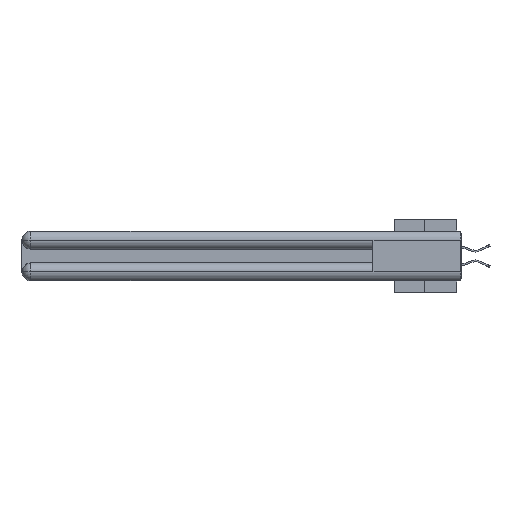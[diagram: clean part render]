
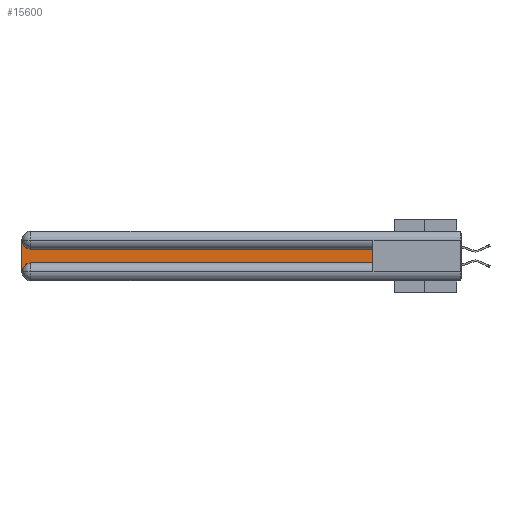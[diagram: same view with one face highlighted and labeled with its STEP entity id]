
A CAD part, left-side view. The second image highlights one B-rep face of the part: STEP entity #15600.
In plain terms, the highlighted planar face has unit normal (-1, 0, 0).
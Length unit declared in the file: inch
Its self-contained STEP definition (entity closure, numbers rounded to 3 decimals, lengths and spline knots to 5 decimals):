
#283 = VERTEX_POINT ( 'NONE', #14710 ) ;
#339 = EDGE_CURVE ( 'NONE', #48209, #17066, #15522, .T. ) ;
#643 = DIRECTION ( 'NONE',  ( 0., 0., -1. ) ) ;
#1827 = AXIS2_PLACEMENT_3D ( 'NONE', #17533, #47625, #32470 ) ;
#1992 = CARTESIAN_POINT ( 'NONE',  ( 0.075, 3., -0.0625 ) ) ;
#3666 = CARTESIAN_POINT ( 'NONE',  ( 0.075, 2.94, -0.2175 ) ) ;
#3961 = VERTEX_POINT ( 'NONE', #3666 ) ;
#4577 = CARTESIAN_POINT ( 'NONE',  ( 0.075, 0.6, -0.2175 ) ) ;
#4660 = CARTESIAN_POINT ( 'NONE',  ( 0.075, 0.6, -0.2175 ) ) ;
#5482 = EDGE_CURVE ( 'NONE', #17066, #39747, #42994, .T. ) ;
#9523 = ORIENTED_EDGE ( 'NONE', *, *, #43273, .T. ) ;
#11518 = DIRECTION ( 'NONE',  ( 1., 0., 0. ) ) ;
#12419 = FACE_OUTER_BOUND ( 'NONE', #30139, .T. ) ;
#13751 = VERTEX_POINT ( 'NONE', #4577 ) ;
#14710 = CARTESIAN_POINT ( 'NONE',  ( 0.075, 0.6, -0.1225 ) ) ;
#15522 = CIRCLE ( 'NONE', #20609, 0.06 ) ;
#15600 = ADVANCED_FACE ( 'NONE', ( #12419 ), #43793, .F. ) ;
#15812 = DIRECTION ( 'NONE',  ( 0., 0., 1. ) ) ;
#17066 = VERTEX_POINT ( 'NONE', #1992 ) ;
#17236 = ORIENTED_EDGE ( 'NONE', *, *, #18871, .T. ) ;
#17533 = CARTESIAN_POINT ( 'NONE',  ( 0.075, 3., -0.1225 ) ) ;
#17558 = CARTESIAN_POINT ( 'NONE',  ( 0.075, 2.94, -0.2775 ) ) ;
#18030 = VECTOR ( 'NONE', #48826, 39.37008 ) ;
#18871 = EDGE_CURVE ( 'NONE', #39747, #3961, #21706, .T. ) ;
#19211 = ORIENTED_EDGE ( 'NONE', *, *, #339, .T. ) ;
#20609 = AXIS2_PLACEMENT_3D ( 'NONE', #34315, #11518, #41828 ) ;
#21706 = CIRCLE ( 'NONE', #27857, 0.06 ) ;
#22790 = VECTOR ( 'NONE', #42804, 39.37008 ) ;
#25052 = DIRECTION ( 'NONE',  ( 0., 0., -1. ) ) ;
#26138 = EDGE_CURVE ( 'NONE', #3961, #13751, #32884, .T. ) ;
#27857 = AXIS2_PLACEMENT_3D ( 'NONE', #17558, #40153, #25052 ) ;
#27937 = CARTESIAN_POINT ( 'NONE',  ( 0.075, 2.94, -0.1225 ) ) ;
#29677 = ORIENTED_EDGE ( 'NONE', *, *, #26138, .T. ) ;
#30139 = EDGE_LOOP ( 'NONE', ( #31979, #19211, #46599, #17236, #29677, #9523 ) ) ;
#31979 = ORIENTED_EDGE ( 'NONE', *, *, #33174, .T. ) ;
#32470 = DIRECTION ( 'NONE',  ( 0., 0., -1. ) ) ;
#32848 = VECTOR ( 'NONE', #643, 39.37008 ) ;
#32884 = LINE ( 'NONE', #38951, #22790 ) ;
#33174 = EDGE_CURVE ( 'NONE', #283, #48209, #38227, .T. ) ;
#34315 = CARTESIAN_POINT ( 'NONE',  ( 0.075, 2.94, -0.0625 ) ) ;
#34841 = VECTOR ( 'NONE', #15812, 39.37008 ) ;
#37894 = CARTESIAN_POINT ( 'NONE',  ( 0.075, 3., -0.2175 ) ) ;
#38227 = LINE ( 'NONE', #40500, #18030 ) ;
#38951 = CARTESIAN_POINT ( 'NONE',  ( 0.075, 0.6, -0.2175 ) ) ;
#39747 = VERTEX_POINT ( 'NONE', #40301 ) ;
#40153 = DIRECTION ( 'NONE',  ( 1., 0., 0. ) ) ;
#40301 = CARTESIAN_POINT ( 'NONE',  ( 0.075, 3., -0.2775 ) ) ;
#40500 = CARTESIAN_POINT ( 'NONE',  ( 0.075, 0.6, -0.1225 ) ) ;
#41828 = DIRECTION ( 'NONE',  ( 0., 0., -1. ) ) ;
#42804 = DIRECTION ( 'NONE',  ( 0., -1., 0. ) ) ;
#42994 = LINE ( 'NONE', #37894, #32848 ) ;
#43273 = EDGE_CURVE ( 'NONE', #13751, #283, #47935, .T. ) ;
#43793 = PLANE ( 'NONE',  #1827 ) ;
#46599 = ORIENTED_EDGE ( 'NONE', *, *, #5482, .T. ) ;
#47625 = DIRECTION ( 'NONE',  ( 1., 0., 0. ) ) ;
#47935 = LINE ( 'NONE', #4660, #34841 ) ;
#48209 = VERTEX_POINT ( 'NONE', #27937 ) ;
#48826 = DIRECTION ( 'NONE',  ( 0., 1., 0. ) ) ;
